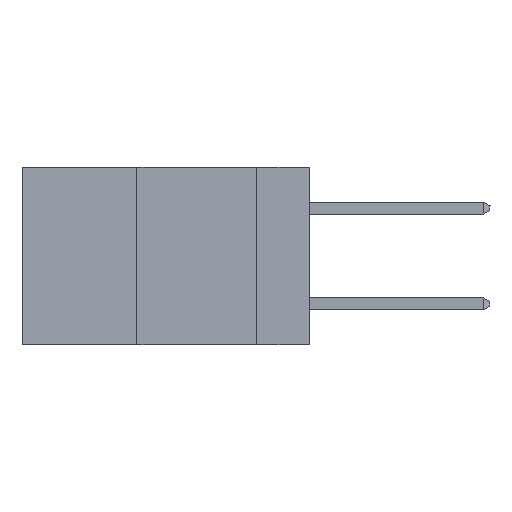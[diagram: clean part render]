
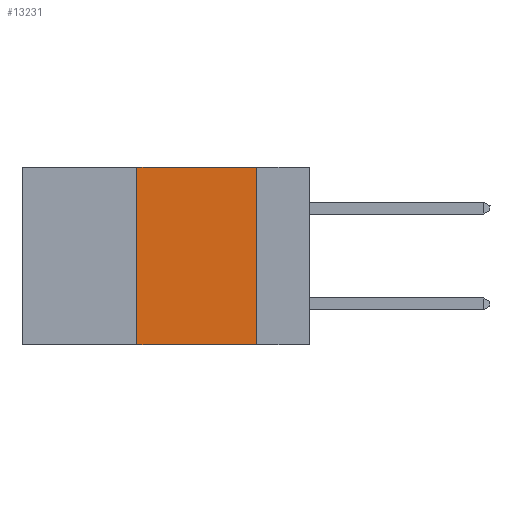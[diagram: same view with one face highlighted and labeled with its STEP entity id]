
A CAD part, left-side view. The second image highlights one B-rep face of the part: STEP entity #13231.
In plain terms, the highlighted planar face has unit normal (-1, 0, 0).
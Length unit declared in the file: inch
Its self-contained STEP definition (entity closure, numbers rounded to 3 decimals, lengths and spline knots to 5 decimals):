
#757 = VECTOR ( 'NONE', #11218, 39.37008 ) ;
#1336 = EDGE_CURVE ( 'NONE', #5188, #12085, #12892, .T. ) ;
#2749 = EDGE_CURVE ( 'NONE', #8264, #12085, #9909, .T. ) ;
#3692 = ORIENTED_EDGE ( 'NONE', *, *, #8321, .F. ) ;
#3956 = CARTESIAN_POINT ( 'NONE',  ( 0., 0.6, -0.37 ) ) ;
#4061 = EDGE_LOOP ( 'NONE', ( #9575, #13058, #3692, #7915 ) ) ;
#4192 = CARTESIAN_POINT ( 'NONE',  ( 0., 0.11, 0. ) ) ;
#4283 = VECTOR ( 'NONE', #12667, 39.37008 ) ;
#4921 = CARTESIAN_POINT ( 'NONE',  ( 0., 0.36, 0. ) ) ;
#5004 = DIRECTION ( 'NONE',  ( 0., -1., 0. ) ) ;
#5188 = VERTEX_POINT ( 'NONE', #4192 ) ;
#5829 = LINE ( 'NONE', #4921, #4283 ) ;
#6468 = DIRECTION ( 'NONE',  ( 0., 0., -1. ) ) ;
#6890 = CARTESIAN_POINT ( 'NONE',  ( 0., 0.36, -0.37 ) ) ;
#6923 = AXIS2_PLACEMENT_3D ( 'NONE', #7458, #10696, #6468 ) ;
#7458 = CARTESIAN_POINT ( 'NONE',  ( 0., 0.6, 0. ) ) ;
#7915 = ORIENTED_EDGE ( 'NONE', *, *, #2749, .T. ) ;
#8264 = VERTEX_POINT ( 'NONE', #6890 ) ;
#8321 = EDGE_CURVE ( 'NONE', #8264, #12095, #5829, .T. ) ;
#9575 = ORIENTED_EDGE ( 'NONE', *, *, #1336, .F. ) ;
#9909 = LINE ( 'NONE', #3956, #14075 ) ;
#10510 = LINE ( 'NONE', #13428, #757 ) ;
#10545 = CARTESIAN_POINT ( 'NONE',  ( 0., 0.11, -0.37 ) ) ;
#10696 = DIRECTION ( 'NONE',  ( 1., 0., 0. ) ) ;
#10788 = PLANE ( 'NONE',  #6923 ) ;
#10938 = DIRECTION ( 'NONE',  ( 0., 0., -1. ) ) ;
#11218 = DIRECTION ( 'NONE',  ( 0., -1., 0. ) ) ;
#11597 = CARTESIAN_POINT ( 'NONE',  ( 0., 0.36, 0. ) ) ;
#11839 = VECTOR ( 'NONE', #10938, 39.37008 ) ;
#12085 = VERTEX_POINT ( 'NONE', #10545 ) ;
#12095 = VERTEX_POINT ( 'NONE', #11597 ) ;
#12667 = DIRECTION ( 'NONE',  ( 0., 0., 1. ) ) ;
#12794 = FACE_OUTER_BOUND ( 'NONE', #4061, .T. ) ;
#12892 = LINE ( 'NONE', #13380, #11839 ) ;
#13058 = ORIENTED_EDGE ( 'NONE', *, *, #13988, .F. ) ;
#13231 = ADVANCED_FACE ( 'NONE', ( #12794 ), #10788, .F. ) ;
#13380 = CARTESIAN_POINT ( 'NONE',  ( 0., 0.11, 0. ) ) ;
#13428 = CARTESIAN_POINT ( 'NONE',  ( 0., 0.6, 0. ) ) ;
#13988 = EDGE_CURVE ( 'NONE', #12095, #5188, #10510, .T. ) ;
#14075 = VECTOR ( 'NONE', #5004, 39.37008 ) ;
